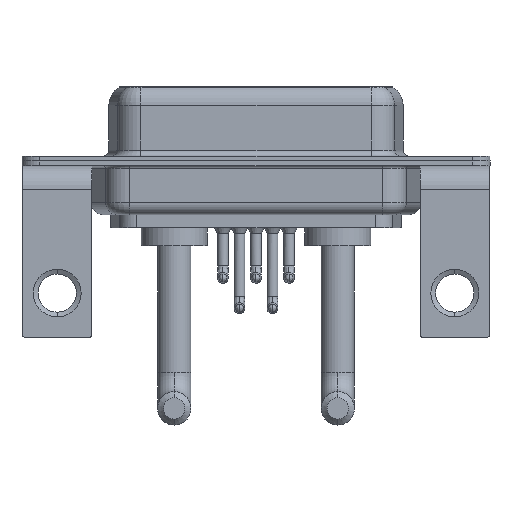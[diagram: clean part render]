
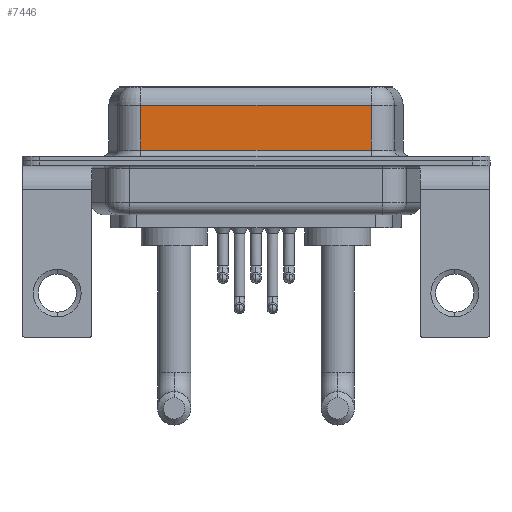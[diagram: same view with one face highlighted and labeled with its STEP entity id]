
A CAD part, front view. The second image highlights one B-rep face of the part: STEP entity #7446.
In plain terms, the highlighted planar face has unit normal (0, -1, 0).
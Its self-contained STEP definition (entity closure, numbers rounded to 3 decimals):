
#175 = CARTESIAN_POINT ( 'NONE',  ( 7.013, -3.95, 0.9 ) ) ;
#628 = CARTESIAN_POINT ( 'NONE',  ( 26.287, -3.95, 0.9 ) ) ;
#1300 = ORIENTED_EDGE ( 'NONE', *, *, #6521, .T. ) ;
#1425 = VERTEX_POINT ( 'NONE', #15214 ) ;
#1618 = DIRECTION ( 'NONE',  ( 0., 0., 1. ) ) ;
#2755 = LINE ( 'NONE', #16125, #14349 ) ;
#3061 = DIRECTION ( 'NONE',  ( 0., 0., -1. ) ) ;
#3443 = LINE ( 'NONE', #8889, #6782 ) ;
#4479 = LINE ( 'NONE', #16953, #9658 ) ;
#4958 = VERTEX_POINT ( 'NONE', #175 ) ;
#5539 = CARTESIAN_POINT ( 'NONE',  ( 7.013, -3.95, 4.65 ) ) ;
#5885 = EDGE_CURVE ( 'NONE', #4958, #12445, #7258, .T. ) ;
#6521 = EDGE_CURVE ( 'NONE', #1425, #12839, #2755, .T. ) ;
#6782 = VECTOR ( 'NONE', #7554, 1000. ) ;
#7258 = LINE ( 'NONE', #14096, #14789 ) ;
#7392 = ORIENTED_EDGE ( 'NONE', *, *, #7928, .T. ) ;
#7446 = ADVANCED_FACE ( 'NONE', ( #12576 ), #15350, .F. ) ;
#7554 = DIRECTION ( 'NONE',  ( 0., 0., -1. ) ) ;
#7928 = EDGE_CURVE ( 'NONE', #12839, #4958, #3443, .T. ) ;
#8330 = EDGE_LOOP ( 'NONE', ( #9882, #1300, #7392, #9522 ) ) ;
#8411 = DIRECTION ( 'NONE',  ( 0., 1., 0. ) ) ;
#8889 = CARTESIAN_POINT ( 'NONE',  ( 7.013, -3.95, 6.4 ) ) ;
#9411 = EDGE_CURVE ( 'NONE', #1425, #12445, #4479, .T. ) ;
#9522 = ORIENTED_EDGE ( 'NONE', *, *, #5885, .T. ) ;
#9658 = VECTOR ( 'NONE', #3061, 1000. ) ;
#9744 = CARTESIAN_POINT ( 'NONE',  ( 26.287, -3.95, 6.4 ) ) ;
#9882 = ORIENTED_EDGE ( 'NONE', *, *, #9411, .F. ) ;
#10096 = DIRECTION ( 'NONE',  ( 1., 0., 0. ) ) ;
#12445 = VERTEX_POINT ( 'NONE', #628 ) ;
#12576 = FACE_OUTER_BOUND ( 'NONE', #8330, .T. ) ;
#12839 = VERTEX_POINT ( 'NONE', #5539 ) ;
#13278 = AXIS2_PLACEMENT_3D ( 'NONE', #9744, #8411, #1618 ) ;
#14096 = CARTESIAN_POINT ( 'NONE',  ( 26.287, -3.95, 0.9 ) ) ;
#14349 = VECTOR ( 'NONE', #15062, 1000. ) ;
#14789 = VECTOR ( 'NONE', #10096, 1000. ) ;
#15062 = DIRECTION ( 'NONE',  ( -1., 0., 0. ) ) ;
#15214 = CARTESIAN_POINT ( 'NONE',  ( 26.287, -3.95, 4.65 ) ) ;
#15350 = PLANE ( 'NONE',  #13278 ) ;
#16125 = CARTESIAN_POINT ( 'NONE',  ( 26.287, -3.95, 4.65 ) ) ;
#16953 = CARTESIAN_POINT ( 'NONE',  ( 26.287, -3.95, 6.4 ) ) ;
